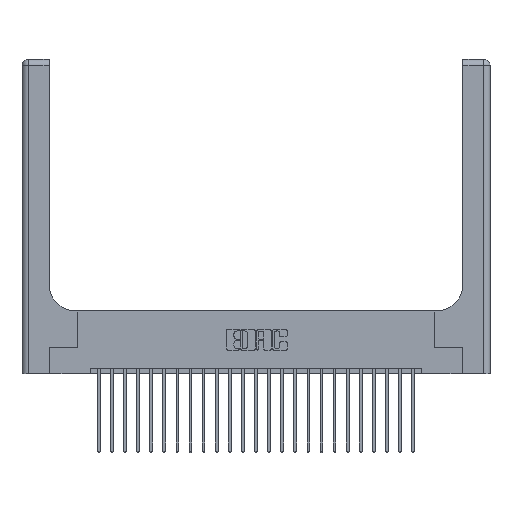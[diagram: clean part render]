
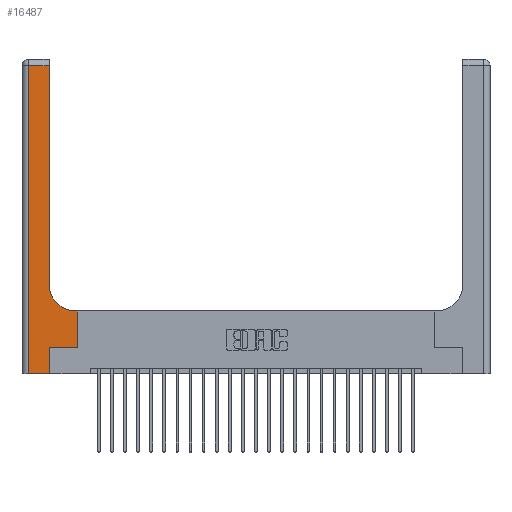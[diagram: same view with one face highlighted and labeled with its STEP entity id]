
A CAD part, top view. The second image highlights one B-rep face of the part: STEP entity #16487.
In plain terms, the highlighted planar face has unit normal (0, 0, 1).
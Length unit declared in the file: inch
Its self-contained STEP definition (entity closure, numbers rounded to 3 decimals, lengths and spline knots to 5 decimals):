
#50 = CARTESIAN_POINT ( 'NONE',  ( 0.26, 0.6, 0.37 ) ) ;
#442 = ORIENTED_EDGE ( 'NONE', *, *, #21423, .T. ) ;
#729 = EDGE_CURVE ( 'NONE', #22279, #10689, #5410, .T. ) ;
#1065 = CARTESIAN_POINT ( 'NONE',  ( 0., 2.94, 0.37 ) ) ;
#1085 = ORIENTED_EDGE ( 'NONE', *, *, #1457, .T. ) ;
#1457 = EDGE_CURVE ( 'NONE', #12135, #3383, #5925, .T. ) ;
#2021 = LINE ( 'NONE', #9527, #16411 ) ;
#2047 = VERTEX_POINT ( 'NONE', #3381 ) ;
#2186 = ORIENTED_EDGE ( 'NONE', *, *, #15773, .T. ) ;
#2230 = CARTESIAN_POINT ( 'NONE',  ( 0.06, 3., 0.37 ) ) ;
#2266 = VERTEX_POINT ( 'NONE', #4698 ) ;
#2579 = VECTOR ( 'NONE', #5359, 39.37008 ) ;
#3381 = CARTESIAN_POINT ( 'NONE',  ( 0.265, 0.25, 0.37 ) ) ;
#3383 = VERTEX_POINT ( 'NONE', #3715 ) ;
#3715 = CARTESIAN_POINT ( 'NONE',  ( 0.06, 2.94, 0.37 ) ) ;
#3805 = VECTOR ( 'NONE', #15623, 39.37008 ) ;
#3898 = AXIS2_PLACEMENT_3D ( 'NONE', #20476, #15155, #13116 ) ;
#4268 = DIRECTION ( 'NONE',  ( 0., -1., 0. ) ) ;
#4277 = CARTESIAN_POINT ( 'NONE',  ( 0.51, 0.6, 0.37 ) ) ;
#4479 = VERTEX_POINT ( 'NONE', #23577 ) ;
#4698 = CARTESIAN_POINT ( 'NONE',  ( 0.06, 0., 0.37 ) ) ;
#4727 = LINE ( 'NONE', #8379, #21698 ) ;
#5202 = EDGE_CURVE ( 'NONE', #4479, #2047, #4727, .T. ) ;
#5359 = DIRECTION ( 'NONE',  ( 1., 0., 0. ) ) ;
#5410 = CIRCLE ( 'NONE', #13512, 0.25 ) ;
#5925 = LINE ( 'NONE', #1065, #12531 ) ;
#6340 = EDGE_LOOP ( 'NONE', ( #11513, #1085, #9674, #6879, #14851, #442, #14633, #2186, #9856 ) ) ;
#6367 = EDGE_CURVE ( 'NONE', #8034, #8153, #23354, .T. ) ;
#6879 = ORIENTED_EDGE ( 'NONE', *, *, #19017, .T. ) ;
#7127 = EDGE_CURVE ( 'NONE', #10689, #12135, #12975, .T. ) ;
#7853 = EDGE_CURVE ( 'NONE', #3383, #2266, #14381, .T. ) ;
#8034 = VERTEX_POINT ( 'NONE', #17808 ) ;
#8153 = VERTEX_POINT ( 'NONE', #23425 ) ;
#8379 = CARTESIAN_POINT ( 'NONE',  ( 0.265, 0., 0.37 ) ) ;
#8778 = DIRECTION ( 'NONE',  ( 1., 0., 0. ) ) ;
#9527 = CARTESIAN_POINT ( 'NONE',  ( 0., 0., 0.37 ) ) ;
#9674 = ORIENTED_EDGE ( 'NONE', *, *, #7853, .T. ) ;
#9856 = ORIENTED_EDGE ( 'NONE', *, *, #729, .T. ) ;
#10070 = LINE ( 'NONE', #14563, #2579 ) ;
#10689 = VERTEX_POINT ( 'NONE', #13946 ) ;
#11513 = ORIENTED_EDGE ( 'NONE', *, *, #7127, .T. ) ;
#12135 = VERTEX_POINT ( 'NONE', #14569 ) ;
#12531 = VECTOR ( 'NONE', #20967, 39.37008 ) ;
#12975 = LINE ( 'NONE', #19951, #19922 ) ;
#13116 = DIRECTION ( 'NONE',  ( -1., 0., 0. ) ) ;
#13360 = PLANE ( 'NONE',  #3898 ) ;
#13512 = AXIS2_PLACEMENT_3D ( 'NONE', #23397, #14205, #8778 ) ;
#13534 = CARTESIAN_POINT ( 'NONE',  ( 0.528, 0.25, 0.37 ) ) ;
#13916 = LINE ( 'NONE', #50, #17944 ) ;
#13946 = CARTESIAN_POINT ( 'NONE',  ( 0.26, 0.85, 0.37 ) ) ;
#14205 = DIRECTION ( 'NONE',  ( 0., 0., -1. ) ) ;
#14381 = LINE ( 'NONE', #2230, #21888 ) ;
#14563 = CARTESIAN_POINT ( 'NONE',  ( 0.265, 0.25, 0.37 ) ) ;
#14569 = CARTESIAN_POINT ( 'NONE',  ( 0.26, 2.94, 0.37 ) ) ;
#14633 = ORIENTED_EDGE ( 'NONE', *, *, #6367, .T. ) ;
#14851 = ORIENTED_EDGE ( 'NONE', *, *, #5202, .T. ) ;
#15155 = DIRECTION ( 'NONE',  ( 0., 0., -1. ) ) ;
#15623 = DIRECTION ( 'NONE',  ( 0., 1., 0. ) ) ;
#15773 = EDGE_CURVE ( 'NONE', #8153, #22279, #13916, .T. ) ;
#16411 = VECTOR ( 'NONE', #17057, 39.37008 ) ;
#16467 = DIRECTION ( 'NONE',  ( -1., 0., 0. ) ) ;
#16487 = ADVANCED_FACE ( 'NONE', ( #16488 ), #13360, .F. ) ;
#16488 = FACE_OUTER_BOUND ( 'NONE', #6340, .T. ) ;
#17057 = DIRECTION ( 'NONE',  ( 1., 0., 0. ) ) ;
#17516 = DIRECTION ( 'NONE',  ( 0., 1., 0. ) ) ;
#17808 = CARTESIAN_POINT ( 'NONE',  ( 0.528, 0.25, 0.37 ) ) ;
#17944 = VECTOR ( 'NONE', #16467, 39.37008 ) ;
#18383 = DIRECTION ( 'NONE',  ( 0., 1., 0. ) ) ;
#19017 = EDGE_CURVE ( 'NONE', #2266, #4479, #2021, .T. ) ;
#19922 = VECTOR ( 'NONE', #18383, 39.37008 ) ;
#19951 = CARTESIAN_POINT ( 'NONE',  ( 0.26, 3., 0.37 ) ) ;
#20476 = CARTESIAN_POINT ( 'NONE',  ( 0., 3., 0.37 ) ) ;
#20967 = DIRECTION ( 'NONE',  ( -1., 0., 0. ) ) ;
#21423 = EDGE_CURVE ( 'NONE', #2047, #8034, #10070, .T. ) ;
#21698 = VECTOR ( 'NONE', #17516, 39.37008 ) ;
#21888 = VECTOR ( 'NONE', #4268, 39.37008 ) ;
#22279 = VERTEX_POINT ( 'NONE', #4277 ) ;
#23354 = LINE ( 'NONE', #13534, #3805 ) ;
#23397 = CARTESIAN_POINT ( 'NONE',  ( 0.51, 0.85, 0.37 ) ) ;
#23425 = CARTESIAN_POINT ( 'NONE',  ( 0.528, 0.6, 0.37 ) ) ;
#23577 = CARTESIAN_POINT ( 'NONE',  ( 0.265, 0., 0.37 ) ) ;
